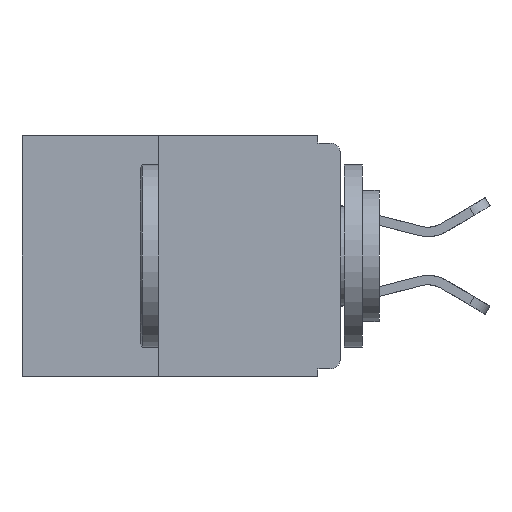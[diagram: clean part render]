
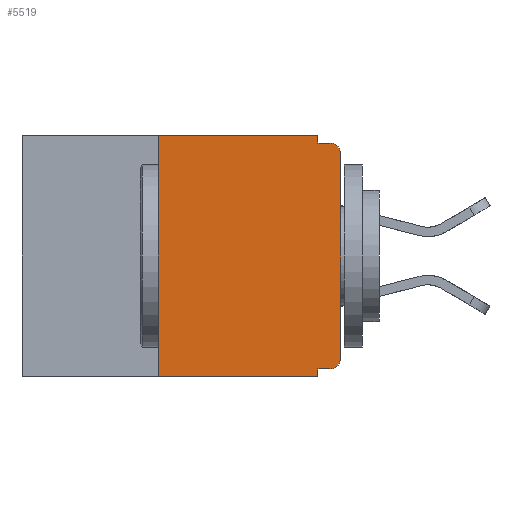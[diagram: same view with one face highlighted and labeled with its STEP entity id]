
A CAD part, left-side view. The second image highlights one B-rep face of the part: STEP entity #5519.
In plain terms, the highlighted planar face has unit normal (-1, 0, 0).
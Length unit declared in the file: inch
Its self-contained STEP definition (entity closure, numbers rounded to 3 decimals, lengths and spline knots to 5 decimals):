
#69 = CARTESIAN_POINT ( 'NONE',  ( 0., 0.015, -0.01 ) ) ;
#199 = EDGE_CURVE ( 'NONE', #26604, #9681, #7445, .T. ) ;
#833 = CARTESIAN_POINT ( 'NONE',  ( 0., 0., -0.01 ) ) ;
#1841 = VERTEX_POINT ( 'NONE', #11970 ) ;
#2028 = LINE ( 'NONE', #13704, #21583 ) ;
#2036 = LINE ( 'NONE', #4454, #7263 ) ;
#2395 = DIRECTION ( 'NONE',  ( 0., 1., 0. ) ) ;
#2503 = CARTESIAN_POINT ( 'NONE',  ( 0., 0., -0.32 ) ) ;
#2823 = ORIENTED_EDGE ( 'NONE', *, *, #27929, .F. ) ;
#2831 = CARTESIAN_POINT ( 'NONE',  ( 0., 0.031, -0.01 ) ) ;
#3150 = CARTESIAN_POINT ( 'NONE',  ( 0., 0.015, -0.305 ) ) ;
#3189 = ORIENTED_EDGE ( 'NONE', *, *, #28717, .F. ) ;
#3409 = DIRECTION ( 'NONE',  ( 0., -1., 0. ) ) ;
#4149 = EDGE_CURVE ( 'NONE', #14651, #17433, #18350, .T. ) ;
#4454 = CARTESIAN_POINT ( 'NONE',  ( 0., 0.437, -0.33 ) ) ;
#4733 = CIRCLE ( 'NONE', #15981, 0.015 ) ;
#5264 = EDGE_CURVE ( 'NONE', #1841, #13538, #11102, .T. ) ;
#5421 = ORIENTED_EDGE ( 'NONE', *, *, #17888, .T. ) ;
#5519 = ADVANCED_FACE ( 'NONE', ( #9566 ), #32708, .F. ) ;
#5745 = DIRECTION ( 'NONE',  ( 0., 0., -1. ) ) ;
#6433 = AXIS2_PLACEMENT_3D ( 'NONE', #25338, #25299, #25265 ) ;
#6537 = VERTEX_POINT ( 'NONE', #15095 ) ;
#6906 = EDGE_CURVE ( 'NONE', #8028, #14651, #14667, .T. ) ;
#7161 = ORIENTED_EDGE ( 'NONE', *, *, #31393, .F. ) ;
#7204 = ORIENTED_EDGE ( 'NONE', *, *, #5264, .F. ) ;
#7263 = VECTOR ( 'NONE', #22284, 39.37008 ) ;
#7445 = LINE ( 'NONE', #27060, #13440 ) ;
#7958 = ORIENTED_EDGE ( 'NONE', *, *, #199, .F. ) ;
#8028 = VERTEX_POINT ( 'NONE', #28773 ) ;
#9394 = CARTESIAN_POINT ( 'NONE',  ( 0., 0.031, -0.33 ) ) ;
#9566 = FACE_OUTER_BOUND ( 'NONE', #29595, .T. ) ;
#9581 = CARTESIAN_POINT ( 'NONE',  ( 0., 0.25, -0.33 ) ) ;
#9681 = VERTEX_POINT ( 'NONE', #9394 ) ;
#10320 = VECTOR ( 'NONE', #24799, 39.37008 ) ;
#10416 = CARTESIAN_POINT ( 'NONE',  ( 0., 0.031, -0.32 ) ) ;
#11102 = LINE ( 'NONE', #24287, #10320 ) ;
#11970 = CARTESIAN_POINT ( 'NONE',  ( 0., 0.031, 0. ) ) ;
#12182 = VERTEX_POINT ( 'NONE', #28161 ) ;
#13066 = LINE ( 'NONE', #833, #32508 ) ;
#13440 = VECTOR ( 'NONE', #24506, 39.37008 ) ;
#13538 = VERTEX_POINT ( 'NONE', #2831 ) ;
#13571 = ORIENTED_EDGE ( 'NONE', *, *, #29778, .T. ) ;
#13704 = CARTESIAN_POINT ( 'NONE',  ( 0., 0.25, -0.33 ) ) ;
#13859 = VECTOR ( 'NONE', #16719, 39.37008 ) ;
#14651 = VERTEX_POINT ( 'NONE', #27775 ) ;
#14667 = LINE ( 'NONE', #19116, #13859 ) ;
#15095 = CARTESIAN_POINT ( 'NONE',  ( 0., 0.25, 0. ) ) ;
#15981 = AXIS2_PLACEMENT_3D ( 'NONE', #3150, #20981, #5745 ) ;
#16719 = DIRECTION ( 'NONE',  ( 0., 0., 1. ) ) ;
#16939 = ORIENTED_EDGE ( 'NONE', *, *, #4149, .T. ) ;
#16978 = LINE ( 'NONE', #2503, #28913 ) ;
#17433 = VERTEX_POINT ( 'NONE', #69 ) ;
#17888 = EDGE_CURVE ( 'NONE', #31247, #9681, #2036, .T. ) ;
#18350 = CIRCLE ( 'NONE', #6433, 0.015 ) ;
#19116 = CARTESIAN_POINT ( 'NONE',  ( 0., 0., 0. ) ) ;
#20981 = DIRECTION ( 'NONE',  ( -1., 0., 0. ) ) ;
#21583 = VECTOR ( 'NONE', #31459, 39.37008 ) ;
#21762 = CARTESIAN_POINT ( 'NONE',  ( 0., 0.437, 0. ) ) ;
#21769 = CARTESIAN_POINT ( 'NONE',  ( 0., 0.437, 0. ) ) ;
#22284 = DIRECTION ( 'NONE',  ( 0., -1., 0. ) ) ;
#23959 = LINE ( 'NONE', #21762, #29110 ) ;
#24287 = CARTESIAN_POINT ( 'NONE',  ( 0., 0.031, 0. ) ) ;
#24506 = DIRECTION ( 'NONE',  ( 0., 0., -1. ) ) ;
#24799 = DIRECTION ( 'NONE',  ( 0., 0., -1. ) ) ;
#25265 = DIRECTION ( 'NONE',  ( 0., 0., -1. ) ) ;
#25299 = DIRECTION ( 'NONE',  ( -1., 0., 0. ) ) ;
#25338 = CARTESIAN_POINT ( 'NONE',  ( 0., 0.015, -0.025 ) ) ;
#25697 = EDGE_CURVE ( 'NONE', #13538, #17433, #13066, .T. ) ;
#26604 = VERTEX_POINT ( 'NONE', #10416 ) ;
#27060 = CARTESIAN_POINT ( 'NONE',  ( 0., 0.031, -0.33 ) ) ;
#27775 = CARTESIAN_POINT ( 'NONE',  ( 0., 0., -0.025 ) ) ;
#27824 = AXIS2_PLACEMENT_3D ( 'NONE', #21769, #32663, #32595 ) ;
#27929 = EDGE_CURVE ( 'NONE', #31247, #6537, #2028, .T. ) ;
#28161 = CARTESIAN_POINT ( 'NONE',  ( 0., 0.015, -0.32 ) ) ;
#28717 = EDGE_CURVE ( 'NONE', #6537, #1841, #23959, .T. ) ;
#28773 = CARTESIAN_POINT ( 'NONE',  ( 0., 0., -0.305 ) ) ;
#28913 = VECTOR ( 'NONE', #2395, 39.37008 ) ;
#29110 = VECTOR ( 'NONE', #29446, 39.37008 ) ;
#29446 = DIRECTION ( 'NONE',  ( 0., -1., 0. ) ) ;
#29595 = EDGE_LOOP ( 'NONE', ( #30940, #16939, #32056, #7204, #3189, #2823, #5421, #7958, #7161, #13571 ) ) ;
#29778 = EDGE_CURVE ( 'NONE', #12182, #8028, #4733, .T. ) ;
#30940 = ORIENTED_EDGE ( 'NONE', *, *, #6906, .T. ) ;
#31247 = VERTEX_POINT ( 'NONE', #9581 ) ;
#31393 = EDGE_CURVE ( 'NONE', #12182, #26604, #16978, .T. ) ;
#31459 = DIRECTION ( 'NONE',  ( 0., 0., 1. ) ) ;
#32056 = ORIENTED_EDGE ( 'NONE', *, *, #25697, .F. ) ;
#32508 = VECTOR ( 'NONE', #3409, 39.37008 ) ;
#32595 = DIRECTION ( 'NONE',  ( 0., 0., -1. ) ) ;
#32663 = DIRECTION ( 'NONE',  ( 1., 0., 0. ) ) ;
#32708 = PLANE ( 'NONE',  #27824 ) ;
